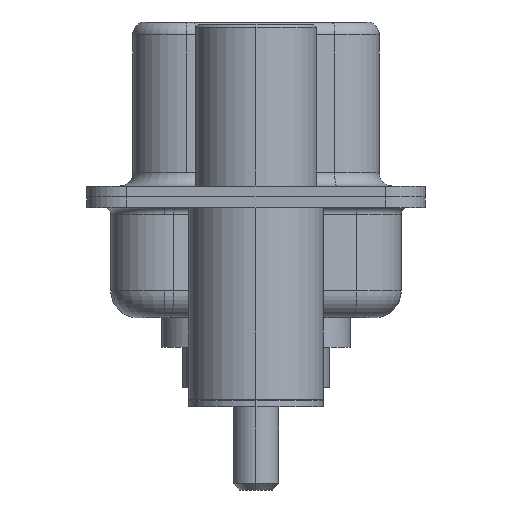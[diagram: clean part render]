
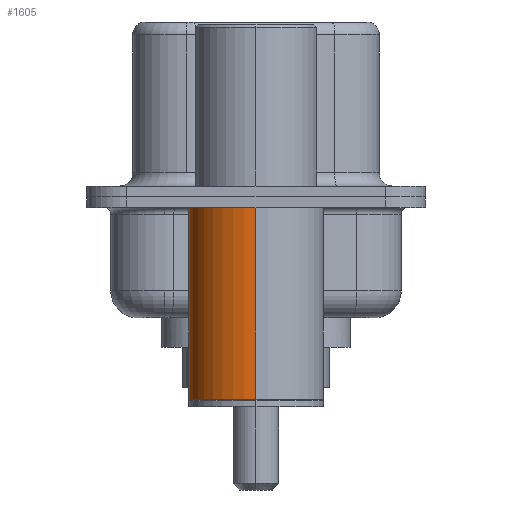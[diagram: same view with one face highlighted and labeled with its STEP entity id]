
A CAD part, left-side view. The second image highlights one B-rep face of the part: STEP entity #1605.
In plain terms, the highlighted cylindrical face has radius 2.5 mm (diameter 5 mm), a partial arc.
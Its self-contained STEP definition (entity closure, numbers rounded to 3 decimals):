
#866 = ORIENTED_EDGE ( 'NONE', *, *, #2634, .F. ) ;
#877 = CARTESIAN_POINT ( 'NONE',  ( 2.5, 0., -7.525 ) ) ;
#1057 = CARTESIAN_POINT ( 'NONE',  ( -2.5, 0., -7.525 ) ) ;
#1605 = ADVANCED_FACE ( 'NONE', ( #13269 ), #3198, .T. ) ;
#1608 = DIRECTION ( 'NONE',  ( 0., 0., 1. ) ) ;
#1814 = EDGE_CURVE ( 'NONE', #3687, #13214, #13459, .T. ) ;
#2634 = EDGE_CURVE ( 'NONE', #13214, #13764, #9045, .T. ) ;
#3063 = ORIENTED_EDGE ( 'NONE', *, *, #3994, .T. ) ;
#3198 = CYLINDRICAL_SURFACE ( 'NONE', #14174, 2.5 ) ;
#3687 = VERTEX_POINT ( 'NONE', #877 ) ;
#3788 = CARTESIAN_POINT ( 'NONE',  ( 0., 0., -0.4 ) ) ;
#3915 = DIRECTION ( 'NONE',  ( 1., 0., 0. ) ) ;
#3945 = CARTESIAN_POINT ( 'NONE',  ( -2.5, 0., -0.4 ) ) ;
#3994 = EDGE_CURVE ( 'NONE', #12932, #13764, #6308, .T. ) ;
#5141 = CIRCLE ( 'NONE', #6916, 2.5 ) ;
#5160 = DIRECTION ( 'NONE',  ( 0., 0., 1. ) ) ;
#5490 = EDGE_CURVE ( 'NONE', #3687, #12932, #5141, .T. ) ;
#6308 = LINE ( 'NONE', #11871, #12276 ) ;
#6370 = CARTESIAN_POINT ( 'NONE',  ( 0., 0., 0.581 ) ) ;
#6916 = AXIS2_PLACEMENT_3D ( 'NONE', #9112, #1608, #10417 ) ;
#8199 = DIRECTION ( 'NONE',  ( 0., 0., 1. ) ) ;
#8886 = DIRECTION ( 'NONE',  ( 1., 0., 0. ) ) ;
#9045 = CIRCLE ( 'NONE', #11569, 2.5 ) ;
#9112 = CARTESIAN_POINT ( 'NONE',  ( 0., 0., -7.525 ) ) ;
#9237 = CARTESIAN_POINT ( 'NONE',  ( 2.5, 0., -0.4 ) ) ;
#9663 = VECTOR ( 'NONE', #5160, 1000. ) ;
#10109 = DIRECTION ( 'NONE',  ( 0., 0., 1. ) ) ;
#10152 = EDGE_LOOP ( 'NONE', ( #13890, #3063, #866, #13543 ) ) ;
#10417 = DIRECTION ( 'NONE',  ( 1., 0., 0. ) ) ;
#11569 = AXIS2_PLACEMENT_3D ( 'NONE', #3788, #8199, #8886 ) ;
#11746 = DIRECTION ( 'NONE',  ( 0., 0., 1. ) ) ;
#11871 = CARTESIAN_POINT ( 'NONE',  ( -2.5, 0., 0.581 ) ) ;
#12276 = VECTOR ( 'NONE', #11746, 1000. ) ;
#12932 = VERTEX_POINT ( 'NONE', #1057 ) ;
#13214 = VERTEX_POINT ( 'NONE', #9237 ) ;
#13269 = FACE_OUTER_BOUND ( 'NONE', #10152, .T. ) ;
#13459 = LINE ( 'NONE', #15855, #9663 ) ;
#13543 = ORIENTED_EDGE ( 'NONE', *, *, #1814, .F. ) ;
#13764 = VERTEX_POINT ( 'NONE', #3945 ) ;
#13890 = ORIENTED_EDGE ( 'NONE', *, *, #5490, .T. ) ;
#14174 = AXIS2_PLACEMENT_3D ( 'NONE', #6370, #10109, #3915 ) ;
#15855 = CARTESIAN_POINT ( 'NONE',  ( 2.5, 0., 0.581 ) ) ;
